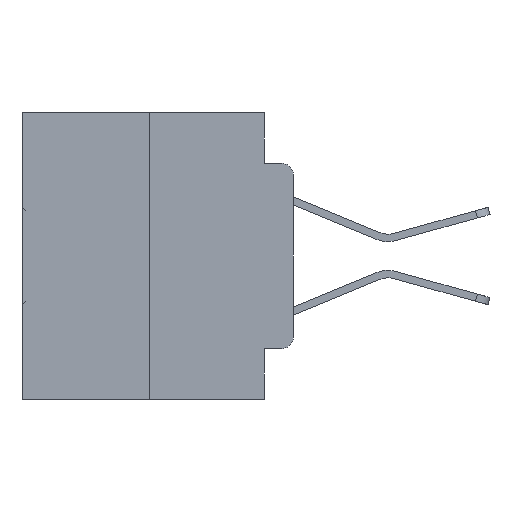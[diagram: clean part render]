
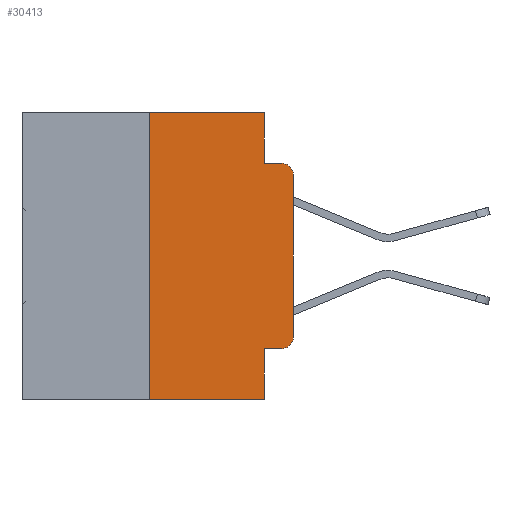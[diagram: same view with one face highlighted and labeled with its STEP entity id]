
A CAD part, left-side view. The second image highlights one B-rep face of the part: STEP entity #30413.
In plain terms, the highlighted planar face has unit normal (-1, 0, 0).
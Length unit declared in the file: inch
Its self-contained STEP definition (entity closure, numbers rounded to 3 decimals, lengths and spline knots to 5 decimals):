
#288 = CARTESIAN_POINT ( 'NONE',  ( 0., 0.051, -0.5 ) ) ;
#635 = CARTESIAN_POINT ( 'NONE',  ( 0., 0.02, -0.0885 ) ) ;
#1319 = VECTOR ( 'NONE', #28233, 39.37008 ) ;
#1619 = AXIS2_PLACEMENT_3D ( 'NONE', #33274, #19797, #30223 ) ;
#1790 = EDGE_CURVE ( 'NONE', #15433, #19202, #23788, .T. ) ;
#2893 = VECTOR ( 'NONE', #21459, 39.37008 ) ;
#2902 = VERTEX_POINT ( 'NONE', #288 ) ;
#3330 = ORIENTED_EDGE ( 'NONE', *, *, #28064, .F. ) ;
#3533 = DIRECTION ( 'NONE',  ( 0., -1., 0. ) ) ;
#5261 = CARTESIAN_POINT ( 'NONE',  ( 0., 0.473, 0. ) ) ;
#5397 = EDGE_CURVE ( 'NONE', #30161, #29200, #20110, .T. ) ;
#5603 = VECTOR ( 'NONE', #3533, 39.37008 ) ;
#5783 = CIRCLE ( 'NONE', #33499, 0.02 ) ;
#6334 = VERTEX_POINT ( 'NONE', #25453 ) ;
#6434 = CARTESIAN_POINT ( 'NONE',  ( 0., 0.02, -0.1085 ) ) ;
#7648 = ORIENTED_EDGE ( 'NONE', *, *, #12593, .F. ) ;
#7764 = CARTESIAN_POINT ( 'NONE',  ( 0., 0.051, 0. ) ) ;
#9425 = FACE_OUTER_BOUND ( 'NONE', #30652, .T. ) ;
#9841 = EDGE_CURVE ( 'NONE', #6334, #12374, #28995, .T. ) ;
#10076 = DIRECTION ( 'NONE',  ( 0., -1., 0. ) ) ;
#10596 = ORIENTED_EDGE ( 'NONE', *, *, #1790, .F. ) ;
#11053 = ORIENTED_EDGE ( 'NONE', *, *, #9841, .F. ) ;
#11086 = CARTESIAN_POINT ( 'NONE',  ( 0., 0.051, -0.0885 ) ) ;
#11092 = EDGE_CURVE ( 'NONE', #15154, #2902, #18156, .T. ) ;
#11660 = VECTOR ( 'NONE', #19336, 39.37008 ) ;
#11685 = ORIENTED_EDGE ( 'NONE', *, *, #12721, .T. ) ;
#11850 = DIRECTION ( 'NONE',  ( -1., 0., 0. ) ) ;
#12374 = VERTEX_POINT ( 'NONE', #635 ) ;
#12593 = EDGE_CURVE ( 'NONE', #19202, #6334, #32155, .T. ) ;
#12721 = EDGE_CURVE ( 'NONE', #16846, #31563, #32996, .T. ) ;
#15154 = VERTEX_POINT ( 'NONE', #31751 ) ;
#15433 = VERTEX_POINT ( 'NONE', #20458 ) ;
#15607 = DIRECTION ( 'NONE',  ( 0., -1., 0. ) ) ;
#16846 = VERTEX_POINT ( 'NONE', #22739 ) ;
#17537 = CARTESIAN_POINT ( 'NONE',  ( 0., 0.051, -0.4115 ) ) ;
#17881 = VECTOR ( 'NONE', #18115, 39.37008 ) ;
#18115 = DIRECTION ( 'NONE',  ( 0., 0., -1. ) ) ;
#18156 = LINE ( 'NONE', #24121, #5603 ) ;
#18183 = ORIENTED_EDGE ( 'NONE', *, *, #23934, .T. ) ;
#18747 = CARTESIAN_POINT ( 'NONE',  ( 0., 0.02, -0.3915 ) ) ;
#19202 = VERTEX_POINT ( 'NONE', #20775 ) ;
#19336 = DIRECTION ( 'NONE',  ( 0., 0., -1. ) ) ;
#19365 = CARTESIAN_POINT ( 'NONE',  ( 0., 0.25, 0. ) ) ;
#19797 = DIRECTION ( 'NONE',  ( 1., 0., 0. ) ) ;
#19978 = PLANE ( 'NONE',  #1619 ) ;
#20110 = LINE ( 'NONE', #17537, #23423 ) ;
#20220 = ORIENTED_EDGE ( 'NONE', *, *, #11092, .T. ) ;
#20230 = ORIENTED_EDGE ( 'NONE', *, *, #26925, .T. ) ;
#20458 = CARTESIAN_POINT ( 'NONE',  ( 0., 0.25, 0. ) ) ;
#20636 = DIRECTION ( 'NONE',  ( 0., 0., -1. ) ) ;
#20775 = CARTESIAN_POINT ( 'NONE',  ( 0., 0.051, 0. ) ) ;
#20902 = AXIS2_PLACEMENT_3D ( 'NONE', #18747, #21490, #31588 ) ;
#21459 = DIRECTION ( 'NONE',  ( 0., -1., 0. ) ) ;
#21490 = DIRECTION ( 'NONE',  ( -1., 0., 0. ) ) ;
#22244 = ORIENTED_EDGE ( 'NONE', *, *, #30143, .F. ) ;
#22739 = CARTESIAN_POINT ( 'NONE',  ( 0., 0., -0.3915 ) ) ;
#22813 = ORIENTED_EDGE ( 'NONE', *, *, #5397, .T. ) ;
#23423 = VECTOR ( 'NONE', #10076, 39.37008 ) ;
#23530 = CARTESIAN_POINT ( 'NONE',  ( 0., 0.02, -0.4115 ) ) ;
#23579 = CARTESIAN_POINT ( 'NONE',  ( 0., 0.051, -0.4115 ) ) ;
#23788 = LINE ( 'NONE', #5261, #24171 ) ;
#23934 = EDGE_CURVE ( 'NONE', #29200, #16846, #30733, .T. ) ;
#24121 = CARTESIAN_POINT ( 'NONE',  ( 0., 0.473, -0.5 ) ) ;
#24171 = VECTOR ( 'NONE', #15607, 39.37008 ) ;
#25453 = CARTESIAN_POINT ( 'NONE',  ( 0., 0.051, -0.0885 ) ) ;
#26343 = CARTESIAN_POINT ( 'NONE',  ( 0., 0., -0.1085 ) ) ;
#26925 = EDGE_CURVE ( 'NONE', #31563, #12374, #5783, .T. ) ;
#28064 = EDGE_CURVE ( 'NONE', #15154, #15433, #32346, .T. ) ;
#28233 = DIRECTION ( 'NONE',  ( 0., 0., 1. ) ) ;
#28995 = LINE ( 'NONE', #11086, #2893 ) ;
#29200 = VERTEX_POINT ( 'NONE', #23530 ) ;
#29244 = VECTOR ( 'NONE', #29808, 39.37008 ) ;
#29599 = CARTESIAN_POINT ( 'NONE',  ( 0., 0.051, 0. ) ) ;
#29808 = DIRECTION ( 'NONE',  ( 0., 0., 1. ) ) ;
#30143 = EDGE_CURVE ( 'NONE', #30161, #2902, #31270, .T. ) ;
#30161 = VERTEX_POINT ( 'NONE', #23579 ) ;
#30223 = DIRECTION ( 'NONE',  ( 0., 0., -1. ) ) ;
#30413 = ADVANCED_FACE ( 'NONE', ( #9425 ), #19978, .F. ) ;
#30610 = CARTESIAN_POINT ( 'NONE',  ( 0., 0., 0. ) ) ;
#30652 = EDGE_LOOP ( 'NONE', ( #11685, #20230, #11053, #7648, #10596, #3330, #20220, #22244, #22813, #18183 ) ) ;
#30733 = CIRCLE ( 'NONE', #20902, 0.02 ) ;
#31270 = LINE ( 'NONE', #7764, #17881 ) ;
#31563 = VERTEX_POINT ( 'NONE', #26343 ) ;
#31588 = DIRECTION ( 'NONE',  ( 0., 0., -1. ) ) ;
#31751 = CARTESIAN_POINT ( 'NONE',  ( 0., 0.25, -0.5 ) ) ;
#32155 = LINE ( 'NONE', #29599, #11660 ) ;
#32346 = LINE ( 'NONE', #19365, #29244 ) ;
#32996 = LINE ( 'NONE', #30610, #1319 ) ;
#33274 = CARTESIAN_POINT ( 'NONE',  ( 0., 0.473, 0. ) ) ;
#33499 = AXIS2_PLACEMENT_3D ( 'NONE', #6434, #11850, #20636 ) ;
